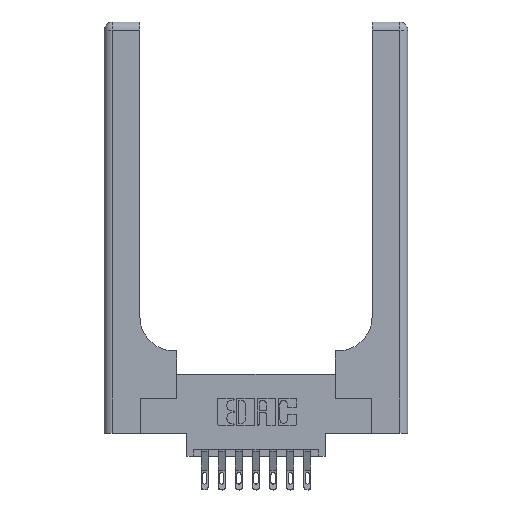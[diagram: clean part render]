
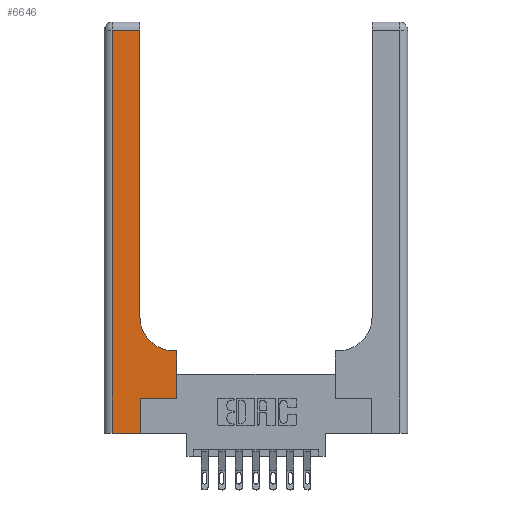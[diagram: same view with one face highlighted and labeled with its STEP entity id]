
A CAD part, top view. The second image highlights one B-rep face of the part: STEP entity #6646.
In plain terms, the highlighted planar face has unit normal (0, 0, 1).
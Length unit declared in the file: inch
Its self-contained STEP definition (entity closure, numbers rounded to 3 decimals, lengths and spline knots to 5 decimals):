
#332 = VERTEX_POINT ( 'NONE', #8314 ) ;
#537 = CARTESIAN_POINT ( 'NONE',  ( 0.265, 0., 0.37 ) ) ;
#801 = CARTESIAN_POINT ( 'NONE',  ( 0.26, 0.6, 0.37 ) ) ;
#975 = DIRECTION ( 'NONE',  ( 0., 0., -1. ) ) ;
#1041 = CIRCLE ( 'NONE', #8741, 0.25 ) ;
#1150 = VERTEX_POINT ( 'NONE', #14117 ) ;
#1447 = CARTESIAN_POINT ( 'NONE',  ( 0.265, 0.25, 0.37 ) ) ;
#1467 = LINE ( 'NONE', #537, #8982 ) ;
#1629 = DIRECTION ( 'NONE',  ( -1., 0., 0. ) ) ;
#1886 = DIRECTION ( 'NONE',  ( -1., 0., 0. ) ) ;
#2227 = LINE ( 'NONE', #4700, #10464 ) ;
#3141 = LINE ( 'NONE', #3981, #14362 ) ;
#3503 = CARTESIAN_POINT ( 'NONE',  ( 0.528, 0.25, 0.37 ) ) ;
#3600 = EDGE_CURVE ( 'NONE', #14715, #14669, #14390, .T. ) ;
#3630 = CARTESIAN_POINT ( 'NONE',  ( 0.51, 0.85, 0.37 ) ) ;
#3828 = VECTOR ( 'NONE', #11617, 39.37008 ) ;
#3981 = CARTESIAN_POINT ( 'NONE',  ( 0., 2.94, 0.37 ) ) ;
#4212 = DIRECTION ( 'NONE',  ( -1., 0., 0. ) ) ;
#4435 = LINE ( 'NONE', #5226, #8242 ) ;
#4471 = DIRECTION ( 'NONE',  ( 0., 1., 0. ) ) ;
#4509 = ORIENTED_EDGE ( 'NONE', *, *, #11071, .T. ) ;
#4532 = CARTESIAN_POINT ( 'NONE',  ( 0., 0., 0.37 ) ) ;
#4700 = CARTESIAN_POINT ( 'NONE',  ( 0.528, 0.25, 0.37 ) ) ;
#4824 = DIRECTION ( 'NONE',  ( 1., 0., 0. ) ) ;
#4967 = EDGE_CURVE ( 'NONE', #1150, #5431, #3141, .T. ) ;
#5202 = PLANE ( 'NONE',  #5259 ) ;
#5226 = CARTESIAN_POINT ( 'NONE',  ( 0.26, 3., 0.37 ) ) ;
#5259 = AXIS2_PLACEMENT_3D ( 'NONE', #9943, #8795, #1629 ) ;
#5431 = VERTEX_POINT ( 'NONE', #6981 ) ;
#5498 = VERTEX_POINT ( 'NONE', #11501 ) ;
#6092 = VECTOR ( 'NONE', #1886, 39.37008 ) ;
#6430 = DIRECTION ( 'NONE',  ( 0., 1., 0. ) ) ;
#6646 = ADVANCED_FACE ( 'NONE', ( #12283 ), #5202, .F. ) ;
#6950 = ORIENTED_EDGE ( 'NONE', *, *, #11272, .T. ) ;
#6981 = CARTESIAN_POINT ( 'NONE',  ( 0.06, 2.94, 0.37 ) ) ;
#7005 = CARTESIAN_POINT ( 'NONE',  ( 0.265, 0.25, 0.37 ) ) ;
#7398 = CARTESIAN_POINT ( 'NONE',  ( 0.06, 0., 0.37 ) ) ;
#7482 = VERTEX_POINT ( 'NONE', #7398 ) ;
#8011 = CARTESIAN_POINT ( 'NONE',  ( 0.06, 3., 0.37 ) ) ;
#8026 = DIRECTION ( 'NONE',  ( 0., 1., 0. ) ) ;
#8242 = VECTOR ( 'NONE', #8026, 39.37008 ) ;
#8295 = EDGE_CURVE ( 'NONE', #7482, #5498, #10431, .T. ) ;
#8314 = CARTESIAN_POINT ( 'NONE',  ( 0.26, 0.85, 0.37 ) ) ;
#8741 = AXIS2_PLACEMENT_3D ( 'NONE', #3630, #975, #9299 ) ;
#8795 = DIRECTION ( 'NONE',  ( 0., 0., -1. ) ) ;
#8982 = VECTOR ( 'NONE', #6430, 39.37008 ) ;
#9299 = DIRECTION ( 'NONE',  ( 1., 0., 0. ) ) ;
#9943 = CARTESIAN_POINT ( 'NONE',  ( 0., 3., 0.37 ) ) ;
#10032 = ORIENTED_EDGE ( 'NONE', *, *, #10432, .T. ) ;
#10262 = VECTOR ( 'NONE', #13740, 39.37008 ) ;
#10431 = LINE ( 'NONE', #4532, #3828 ) ;
#10432 = EDGE_CURVE ( 'NONE', #14669, #12869, #2227, .T. ) ;
#10453 = EDGE_CURVE ( 'NONE', #13537, #332, #1041, .T. ) ;
#10464 = VECTOR ( 'NONE', #4471, 39.37008 ) ;
#10562 = ORIENTED_EDGE ( 'NONE', *, *, #10795, .T. ) ;
#10582 = ORIENTED_EDGE ( 'NONE', *, *, #4967, .T. ) ;
#10795 = EDGE_CURVE ( 'NONE', #332, #1150, #4435, .T. ) ;
#11071 = EDGE_CURVE ( 'NONE', #5498, #14715, #1467, .T. ) ;
#11156 = ORIENTED_EDGE ( 'NONE', *, *, #10453, .T. ) ;
#11272 = EDGE_CURVE ( 'NONE', #5431, #7482, #12814, .T. ) ;
#11456 = ORIENTED_EDGE ( 'NONE', *, *, #8295, .T. ) ;
#11501 = CARTESIAN_POINT ( 'NONE',  ( 0.265, 0., 0.37 ) ) ;
#11617 = DIRECTION ( 'NONE',  ( 1., 0., 0. ) ) ;
#11641 = VECTOR ( 'NONE', #4824, 39.37008 ) ;
#12283 = FACE_OUTER_BOUND ( 'NONE', #13250, .T. ) ;
#12814 = LINE ( 'NONE', #8011, #10262 ) ;
#12869 = VERTEX_POINT ( 'NONE', #13609 ) ;
#12935 = ORIENTED_EDGE ( 'NONE', *, *, #3600, .T. ) ;
#13250 = EDGE_LOOP ( 'NONE', ( #10562, #10582, #6950, #11456, #4509, #12935, #10032, #14682, #11156 ) ) ;
#13537 = VERTEX_POINT ( 'NONE', #14579 ) ;
#13609 = CARTESIAN_POINT ( 'NONE',  ( 0.528, 0.6, 0.37 ) ) ;
#13740 = DIRECTION ( 'NONE',  ( 0., -1., 0. ) ) ;
#14117 = CARTESIAN_POINT ( 'NONE',  ( 0.26, 2.94, 0.37 ) ) ;
#14362 = VECTOR ( 'NONE', #4212, 39.37008 ) ;
#14390 = LINE ( 'NONE', #7005, #11641 ) ;
#14579 = CARTESIAN_POINT ( 'NONE',  ( 0.51, 0.6, 0.37 ) ) ;
#14669 = VERTEX_POINT ( 'NONE', #3503 ) ;
#14682 = ORIENTED_EDGE ( 'NONE', *, *, #15294, .T. ) ;
#14715 = VERTEX_POINT ( 'NONE', #1447 ) ;
#14945 = LINE ( 'NONE', #801, #6092 ) ;
#15294 = EDGE_CURVE ( 'NONE', #12869, #13537, #14945, .T. ) ;
